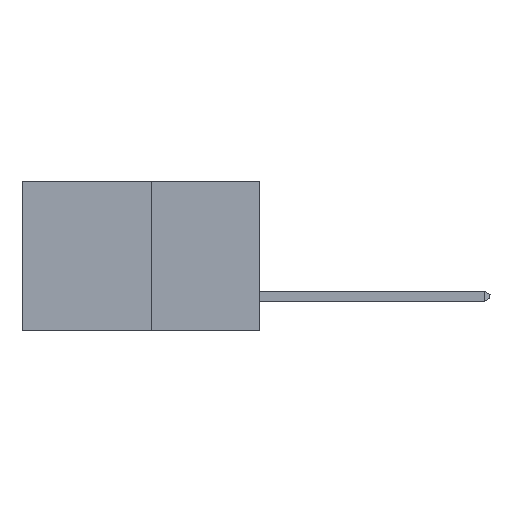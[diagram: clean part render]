
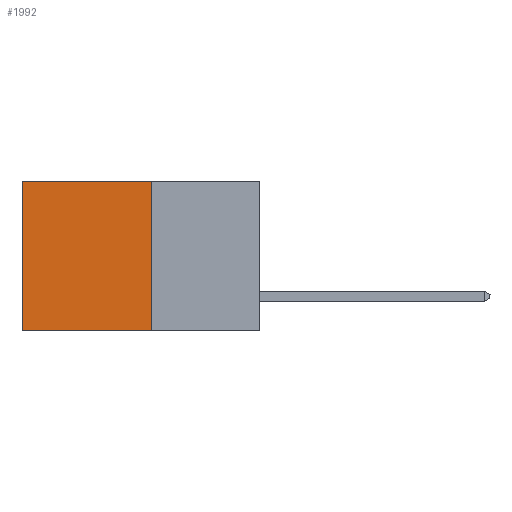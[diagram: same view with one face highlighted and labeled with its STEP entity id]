
A CAD part, left-side view. The second image highlights one B-rep face of the part: STEP entity #1992.
In plain terms, the highlighted planar face has unit normal (-1, 0, 0).
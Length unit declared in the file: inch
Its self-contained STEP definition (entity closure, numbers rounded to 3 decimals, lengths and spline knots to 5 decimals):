
#173 = LINE ( 'NONE', #7533, #6414 ) ;
#244 = CARTESIAN_POINT ( 'NONE',  ( 0.277, 0.59, 0. ) ) ;
#382 = CARTESIAN_POINT ( 'NONE',  ( 0.277, 0.59, -0.37 ) ) ;
#800 = PLANE ( 'NONE',  #8345 ) ;
#1495 = ORIENTED_EDGE ( 'NONE', *, *, #8361, .F. ) ;
#1791 = ORIENTED_EDGE ( 'NONE', *, *, #8696, .T. ) ;
#1992 = ADVANCED_FACE ( 'NONE', ( #6470 ), #800, .F. ) ;
#2114 = CARTESIAN_POINT ( 'NONE',  ( 0.277, 0.27, -0.37 ) ) ;
#2895 = CARTESIAN_POINT ( 'NONE',  ( 0.277, 0.27, 0. ) ) ;
#2941 = VERTEX_POINT ( 'NONE', #7412 ) ;
#2943 = DIRECTION ( 'NONE',  ( 0., 1., 0. ) ) ;
#3590 = ORIENTED_EDGE ( 'NONE', *, *, #9988, .T. ) ;
#4281 = DIRECTION ( 'NONE',  ( 0., 1., 0. ) ) ;
#4282 = VECTOR ( 'NONE', #2943, 39.37008 ) ;
#4363 = VECTOR ( 'NONE', #4281, 39.37008 ) ;
#4673 = VERTEX_POINT ( 'NONE', #9711 ) ;
#4876 = VERTEX_POINT ( 'NONE', #244 ) ;
#4987 = DIRECTION ( 'NONE',  ( 1., 0., 0. ) ) ;
#5006 = DIRECTION ( 'NONE',  ( 0., 0., -1. ) ) ;
#5659 = LINE ( 'NONE', #7317, #9561 ) ;
#5902 = EDGE_LOOP ( 'NONE', ( #1791, #7878, #1495, #3590 ) ) ;
#6293 = DIRECTION ( 'NONE',  ( 0., 0., -1. ) ) ;
#6414 = VECTOR ( 'NONE', #6293, 39.37008 ) ;
#6446 = LINE ( 'NONE', #2895, #4282 ) ;
#6470 = FACE_OUTER_BOUND ( 'NONE', #5902, .T. ) ;
#6949 = DIRECTION ( 'NONE',  ( 0., 0., -1. ) ) ;
#7202 = VERTEX_POINT ( 'NONE', #382 ) ;
#7317 = CARTESIAN_POINT ( 'NONE',  ( 0.277, 0.27, -0.37 ) ) ;
#7412 = CARTESIAN_POINT ( 'NONE',  ( 0.277, 0.27, 0. ) ) ;
#7533 = CARTESIAN_POINT ( 'NONE',  ( 0.277, 0.59, -0.37 ) ) ;
#7878 = ORIENTED_EDGE ( 'NONE', *, *, #9428, .F. ) ;
#8345 = AXIS2_PLACEMENT_3D ( 'NONE', #9069, #4987, #5006 ) ;
#8361 = EDGE_CURVE ( 'NONE', #2941, #4673, #5659, .T. ) ;
#8696 = EDGE_CURVE ( 'NONE', #4876, #7202, #173, .T. ) ;
#9069 = CARTESIAN_POINT ( 'NONE',  ( 0.277, 0.27, -0.37 ) ) ;
#9428 = EDGE_CURVE ( 'NONE', #4673, #7202, #10320, .T. ) ;
#9561 = VECTOR ( 'NONE', #6949, 39.37008 ) ;
#9711 = CARTESIAN_POINT ( 'NONE',  ( 0.277, 0.27, -0.37 ) ) ;
#9988 = EDGE_CURVE ( 'NONE', #2941, #4876, #6446, .T. ) ;
#10320 = LINE ( 'NONE', #2114, #4363 ) ;
